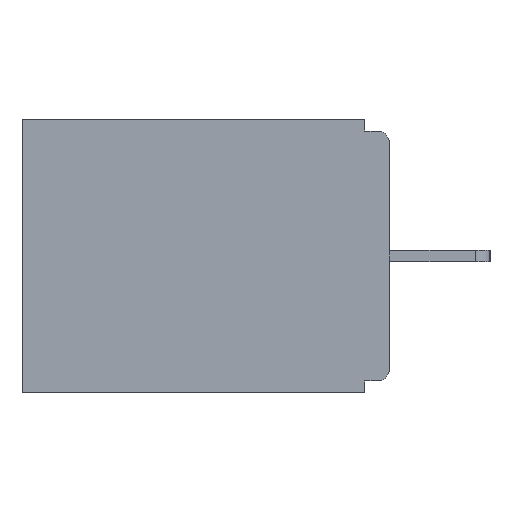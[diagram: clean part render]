
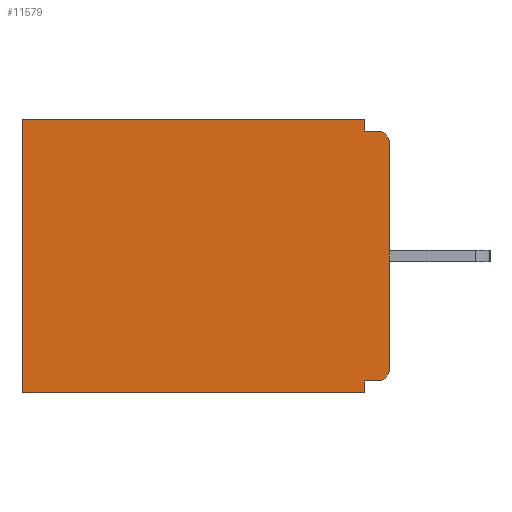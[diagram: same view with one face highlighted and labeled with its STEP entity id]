
A CAD part, left-side view. The second image highlights one B-rep face of the part: STEP entity #11579.
In plain terms, the highlighted planar face has unit normal (-1, 0, 0).
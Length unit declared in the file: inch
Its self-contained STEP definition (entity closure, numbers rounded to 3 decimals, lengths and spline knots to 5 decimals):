
#25 = ORIENTED_EDGE ( 'NONE', *, *, #19186, .F. ) ;
#595 = VECTOR ( 'NONE', #5721, 39.37008 ) ;
#741 = EDGE_CURVE ( 'NONE', #12393, #19573, #18529, .T. ) ;
#907 = VECTOR ( 'NONE', #4586, 39.37008 ) ;
#926 = CARTESIAN_POINT ( 'NONE',  ( 0.298, 0., -0.328 ) ) ;
#959 = VERTEX_POINT ( 'NONE', #8995 ) ;
#1127 = VERTEX_POINT ( 'NONE', #3646 ) ;
#1212 = LINE ( 'NONE', #16574, #5421 ) ;
#2189 = FACE_OUTER_BOUND ( 'NONE', #16495, .T. ) ;
#2219 = EDGE_CURVE ( 'NONE', #1127, #19573, #10239, .T. ) ;
#2333 = AXIS2_PLACEMENT_3D ( 'NONE', #11869, #11830, #3769 ) ;
#2475 = LINE ( 'NONE', #11962, #7127 ) ;
#2705 = EDGE_CURVE ( 'NONE', #9504, #6365, #12754, .T. ) ;
#2745 = DIRECTION ( 'NONE',  ( 0., -1., 0. ) ) ;
#3041 = ORIENTED_EDGE ( 'NONE', *, *, #741, .F. ) ;
#3536 = ORIENTED_EDGE ( 'NONE', *, *, #2219, .T. ) ;
#3646 = CARTESIAN_POINT ( 'NONE',  ( 0.298, 0.46, 0. ) ) ;
#3676 = EDGE_CURVE ( 'NONE', #8407, #15594, #7310, .T. ) ;
#3759 = DIRECTION ( 'NONE',  ( 0., 0., -1. ) ) ;
#3769 = DIRECTION ( 'NONE',  ( 0., 0., -1. ) ) ;
#4123 = ORIENTED_EDGE ( 'NONE', *, *, #11179, .F. ) ;
#4348 = DIRECTION ( 'NONE',  ( 0., 1., 0. ) ) ;
#4586 = DIRECTION ( 'NONE',  ( 0., 1., 0. ) ) ;
#4820 = LINE ( 'NONE', #926, #595 ) ;
#5297 = EDGE_CURVE ( 'NONE', #10824, #11109, #6996, .T. ) ;
#5421 = VECTOR ( 'NONE', #7700, 39.37008 ) ;
#5721 = DIRECTION ( 'NONE',  ( 0., 1., 0. ) ) ;
#5923 = DIRECTION ( 'NONE',  ( -1., 0., 0. ) ) ;
#6075 = CARTESIAN_POINT ( 'NONE',  ( 0.298, 0.015, -0.015 ) ) ;
#6365 = VERTEX_POINT ( 'NONE', #6075 ) ;
#6996 = LINE ( 'NONE', #19299, #14962 ) ;
#7127 = VECTOR ( 'NONE', #2745, 39.37008 ) ;
#7310 = CIRCLE ( 'NONE', #2333, 0.015 ) ;
#7325 = CARTESIAN_POINT ( 'NONE',  ( 0.298, 0., -0.343 ) ) ;
#7361 = CARTESIAN_POINT ( 'NONE',  ( 0.298, 0., 0. ) ) ;
#7700 = DIRECTION ( 'NONE',  ( 0., 0., -1. ) ) ;
#8407 = VERTEX_POINT ( 'NONE', #12517 ) ;
#8868 = DIRECTION ( 'NONE',  ( 0., 0., -1. ) ) ;
#8995 = CARTESIAN_POINT ( 'NONE',  ( 0.298, 0.031, -0.328 ) ) ;
#9060 = AXIS2_PLACEMENT_3D ( 'NONE', #11103, #5923, #9174 ) ;
#9174 = DIRECTION ( 'NONE',  ( 0., 0., -1. ) ) ;
#9260 = VECTOR ( 'NONE', #19169, 39.37008 ) ;
#9504 = VERTEX_POINT ( 'NONE', #12547 ) ;
#9608 = CARTESIAN_POINT ( 'NONE',  ( 0.298, 0., -0.313 ) ) ;
#10068 = AXIS2_PLACEMENT_3D ( 'NONE', #7361, #17731, #8868 ) ;
#10239 = LINE ( 'NONE', #12946, #9260 ) ;
#10703 = VECTOR ( 'NONE', #11810, 39.37008 ) ;
#10824 = VERTEX_POINT ( 'NONE', #18560 ) ;
#11103 = CARTESIAN_POINT ( 'NONE',  ( 0.298, 0.015, -0.03 ) ) ;
#11109 = VERTEX_POINT ( 'NONE', #19317 ) ;
#11159 = LINE ( 'NONE', #19065, #10703 ) ;
#11179 = EDGE_CURVE ( 'NONE', #9504, #15594, #1212, .T. ) ;
#11579 = ADVANCED_FACE ( 'NONE', ( #2189 ), #14817, .F. ) ;
#11810 = DIRECTION ( 'NONE',  ( 0., 0., -1. ) ) ;
#11830 = DIRECTION ( 'NONE',  ( -1., 0., 0. ) ) ;
#11869 = CARTESIAN_POINT ( 'NONE',  ( 0.298, 0.015, -0.313 ) ) ;
#11962 = CARTESIAN_POINT ( 'NONE',  ( 0.298, 0., -0.015 ) ) ;
#12393 = VERTEX_POINT ( 'NONE', #16850 ) ;
#12517 = CARTESIAN_POINT ( 'NONE',  ( 0.298, 0.015, -0.328 ) ) ;
#12547 = CARTESIAN_POINT ( 'NONE',  ( 0.298, 0., -0.03 ) ) ;
#12754 = CIRCLE ( 'NONE', #9060, 0.015 ) ;
#12946 = CARTESIAN_POINT ( 'NONE',  ( 0.298, 0.46, 0. ) ) ;
#13176 = LINE ( 'NONE', #15127, #907 ) ;
#14452 = ORIENTED_EDGE ( 'NONE', *, *, #3676, .T. ) ;
#14684 = VECTOR ( 'NONE', #4348, 39.37008 ) ;
#14817 = PLANE ( 'NONE',  #10068 ) ;
#14962 = VECTOR ( 'NONE', #3759, 39.37008 ) ;
#14963 = EDGE_CURVE ( 'NONE', #10824, #1127, #13176, .T. ) ;
#15127 = CARTESIAN_POINT ( 'NONE',  ( 0.298, 0., 0. ) ) ;
#15527 = ORIENTED_EDGE ( 'NONE', *, *, #14963, .T. ) ;
#15594 = VERTEX_POINT ( 'NONE', #9608 ) ;
#16429 = EDGE_CURVE ( 'NONE', #8407, #959, #4820, .T. ) ;
#16495 = EDGE_LOOP ( 'NONE', ( #19507, #19163, #18067, #15527, #3536, #3041, #25, #16973, #14452, #4123 ) ) ;
#16574 = CARTESIAN_POINT ( 'NONE',  ( 0.298, 0., 0. ) ) ;
#16850 = CARTESIAN_POINT ( 'NONE',  ( 0.298, 0.031, -0.343 ) ) ;
#16973 = ORIENTED_EDGE ( 'NONE', *, *, #16429, .F. ) ;
#17005 = CARTESIAN_POINT ( 'NONE',  ( 0.298, 0.46, -0.343 ) ) ;
#17731 = DIRECTION ( 'NONE',  ( 1., 0., 0. ) ) ;
#18067 = ORIENTED_EDGE ( 'NONE', *, *, #5297, .F. ) ;
#18529 = LINE ( 'NONE', #7325, #14684 ) ;
#18560 = CARTESIAN_POINT ( 'NONE',  ( 0.298, 0.031, 0. ) ) ;
#18743 = EDGE_CURVE ( 'NONE', #11109, #6365, #2475, .T. ) ;
#19065 = CARTESIAN_POINT ( 'NONE',  ( 0.298, 0.031, -0.343 ) ) ;
#19163 = ORIENTED_EDGE ( 'NONE', *, *, #18743, .F. ) ;
#19169 = DIRECTION ( 'NONE',  ( 0., 0., -1. ) ) ;
#19186 = EDGE_CURVE ( 'NONE', #959, #12393, #11159, .T. ) ;
#19299 = CARTESIAN_POINT ( 'NONE',  ( 0.298, 0.031, -0.343 ) ) ;
#19317 = CARTESIAN_POINT ( 'NONE',  ( 0.298, 0.031, -0.015 ) ) ;
#19507 = ORIENTED_EDGE ( 'NONE', *, *, #2705, .T. ) ;
#19573 = VERTEX_POINT ( 'NONE', #17005 ) ;
